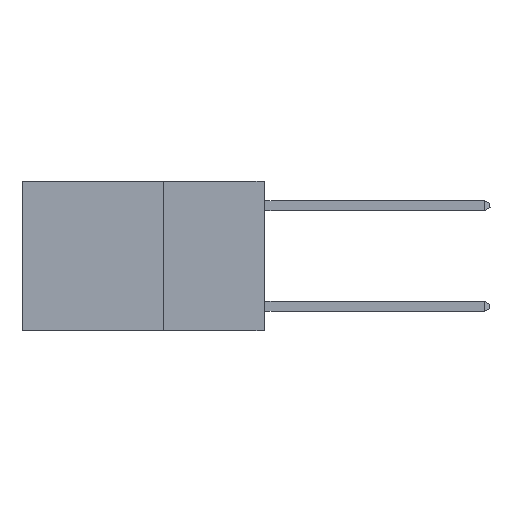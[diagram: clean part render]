
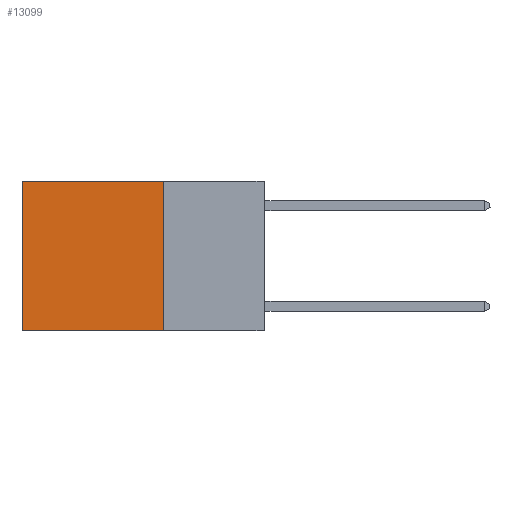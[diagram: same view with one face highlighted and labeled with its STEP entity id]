
A CAD part, left-side view. The second image highlights one B-rep face of the part: STEP entity #13099.
In plain terms, the highlighted planar face has unit normal (-1, 0, 0).
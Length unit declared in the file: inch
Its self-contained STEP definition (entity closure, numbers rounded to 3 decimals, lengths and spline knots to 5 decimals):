
#826 = VERTEX_POINT ( 'NONE', #22668 ) ;
#1192 = EDGE_LOOP ( 'NONE', ( #22703, #21990, #8019, #14607 ) ) ;
#2387 = CARTESIAN_POINT ( 'NONE',  ( 0.2625, 0.25, 0. ) ) ;
#2544 = DIRECTION ( 'NONE',  ( 0., 0., -1. ) ) ;
#3307 = DIRECTION ( 'NONE',  ( 0., 1., 0. ) ) ;
#5064 = CARTESIAN_POINT ( 'NONE',  ( 0.2625, 0.25, -0.37 ) ) ;
#5358 = PLANE ( 'NONE',  #6885 ) ;
#6441 = VECTOR ( 'NONE', #14032, 39.37008 ) ;
#6628 = DIRECTION ( 'NONE',  ( 0., 1., 0. ) ) ;
#6803 = CARTESIAN_POINT ( 'NONE',  ( 0.2625, 0.25, -0.37 ) ) ;
#6885 = AXIS2_PLACEMENT_3D ( 'NONE', #7403, #18252, #7235 ) ;
#7113 = LINE ( 'NONE', #23516, #17739 ) ;
#7235 = DIRECTION ( 'NONE',  ( 0., 0., -1. ) ) ;
#7403 = CARTESIAN_POINT ( 'NONE',  ( 0.2625, 0.25, 0. ) ) ;
#7768 = VERTEX_POINT ( 'NONE', #10410 ) ;
#7883 = LINE ( 'NONE', #12019, #6441 ) ;
#8019 = ORIENTED_EDGE ( 'NONE', *, *, #10352, .F. ) ;
#10352 = EDGE_CURVE ( 'NONE', #7768, #17864, #19250, .T. ) ;
#10410 = CARTESIAN_POINT ( 'NONE',  ( 0.2625, 0.25, 0. ) ) ;
#11376 = VECTOR ( 'NONE', #6628, 39.37008 ) ;
#12019 = CARTESIAN_POINT ( 'NONE',  ( 0.2625, 0.6, 0. ) ) ;
#12027 = EDGE_CURVE ( 'NONE', #7768, #826, #7113, .T. ) ;
#12563 = FACE_OUTER_BOUND ( 'NONE', #1192, .T. ) ;
#13099 = ADVANCED_FACE ( 'NONE', ( #12563 ), #5358, .F. ) ;
#13398 = EDGE_CURVE ( 'NONE', #17864, #22576, #17145, .T. ) ;
#14032 = DIRECTION ( 'NONE',  ( 0., 0., -1. ) ) ;
#14607 = ORIENTED_EDGE ( 'NONE', *, *, #12027, .T. ) ;
#16140 = CARTESIAN_POINT ( 'NONE',  ( 0.2625, 0.6, -0.37 ) ) ;
#16519 = EDGE_CURVE ( 'NONE', #826, #22576, #7883, .T. ) ;
#17145 = LINE ( 'NONE', #6803, #11376 ) ;
#17739 = VECTOR ( 'NONE', #3307, 39.37008 ) ;
#17864 = VERTEX_POINT ( 'NONE', #5064 ) ;
#18252 = DIRECTION ( 'NONE',  ( 1., 0., 0. ) ) ;
#19250 = LINE ( 'NONE', #2387, #20986 ) ;
#20986 = VECTOR ( 'NONE', #2544, 39.37008 ) ;
#21990 = ORIENTED_EDGE ( 'NONE', *, *, #13398, .F. ) ;
#22576 = VERTEX_POINT ( 'NONE', #16140 ) ;
#22668 = CARTESIAN_POINT ( 'NONE',  ( 0.2625, 0.6, 0. ) ) ;
#22703 = ORIENTED_EDGE ( 'NONE', *, *, #16519, .T. ) ;
#23516 = CARTESIAN_POINT ( 'NONE',  ( 0.2625, 0.25, 0. ) ) ;
